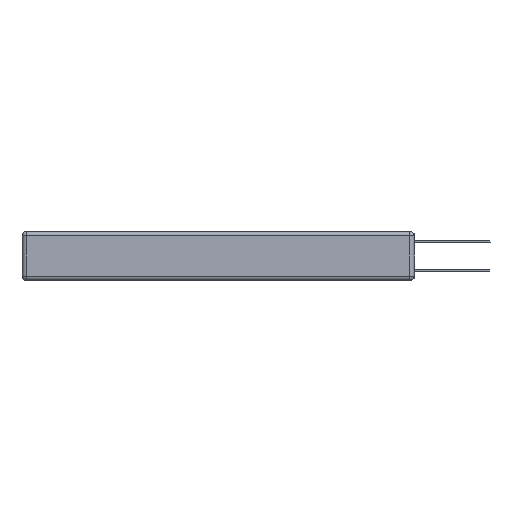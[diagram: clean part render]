
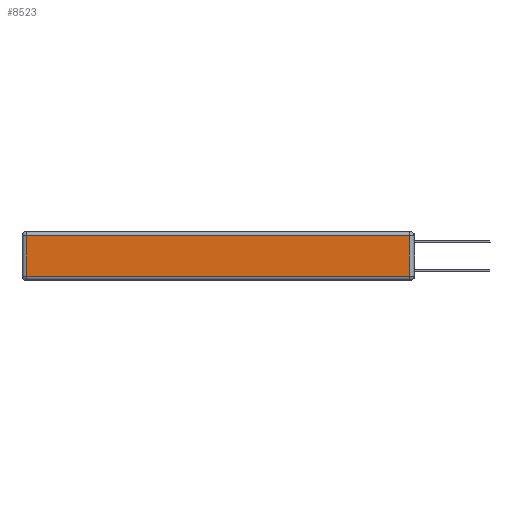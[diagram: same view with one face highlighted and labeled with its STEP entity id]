
A CAD part, left-side view. The second image highlights one B-rep face of the part: STEP entity #8523.
In plain terms, the highlighted planar face has unit normal (-1, 0, 0).
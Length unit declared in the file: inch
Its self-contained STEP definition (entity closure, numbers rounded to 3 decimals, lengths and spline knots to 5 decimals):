
#39 = CARTESIAN_POINT ( 'NONE',  ( 0., 2.72, -0.343 ) ) ;
#441 = VERTEX_POINT ( 'NONE', #12251 ) ;
#1018 = EDGE_CURVE ( 'NONE', #9806, #441, #3056, .T. ) ;
#1954 = EDGE_CURVE ( 'NONE', #6911, #9806, #15482, .T. ) ;
#2604 = VERTEX_POINT ( 'NONE', #8026 ) ;
#2969 = AXIS2_PLACEMENT_3D ( 'NONE', #7080, #16449, #4146 ) ;
#3013 = LINE ( 'NONE', #39, #12522 ) ;
#3056 = LINE ( 'NONE', #7156, #10019 ) ;
#4146 = DIRECTION ( 'NONE',  ( 0., 0., 1. ) ) ;
#5275 = CARTESIAN_POINT ( 'NONE',  ( 0., 0.03, -0.313 ) ) ;
#5506 = EDGE_CURVE ( 'NONE', #2604, #6911, #10618, .T. ) ;
#6911 = VERTEX_POINT ( 'NONE', #5275 ) ;
#7080 = CARTESIAN_POINT ( 'NONE',  ( 0., 0., -0.343 ) ) ;
#7134 = ORIENTED_EDGE ( 'NONE', *, *, #1018, .T. ) ;
#7156 = CARTESIAN_POINT ( 'NONE',  ( 0., 2.75, -0.03 ) ) ;
#7287 = VECTOR ( 'NONE', #13670, 39.37008 ) ;
#8026 = CARTESIAN_POINT ( 'NONE',  ( 0., 2.72, -0.313 ) ) ;
#8049 = FACE_OUTER_BOUND ( 'NONE', #12428, .T. ) ;
#8523 = ADVANCED_FACE ( 'NONE', ( #8049 ), #12398, .T. ) ;
#8541 = ORIENTED_EDGE ( 'NONE', *, *, #5506, .T. ) ;
#8625 = CARTESIAN_POINT ( 'NONE',  ( 0., 0.03, -0.343 ) ) ;
#9091 = CARTESIAN_POINT ( 'NONE',  ( 0., 0.03, -0.03 ) ) ;
#9806 = VERTEX_POINT ( 'NONE', #9091 ) ;
#10019 = VECTOR ( 'NONE', #12945, 39.37008 ) ;
#10618 = LINE ( 'NONE', #17646, #7287 ) ;
#10928 = ORIENTED_EDGE ( 'NONE', *, *, #13962, .T. ) ;
#12251 = CARTESIAN_POINT ( 'NONE',  ( 0., 2.72, -0.03 ) ) ;
#12305 = ORIENTED_EDGE ( 'NONE', *, *, #1954, .T. ) ;
#12398 = PLANE ( 'NONE',  #2969 ) ;
#12428 = EDGE_LOOP ( 'NONE', ( #8541, #12305, #7134, #10928 ) ) ;
#12522 = VECTOR ( 'NONE', #14143, 39.37008 ) ;
#12945 = DIRECTION ( 'NONE',  ( 0., 1., 0. ) ) ;
#13670 = DIRECTION ( 'NONE',  ( 0., -1., 0. ) ) ;
#13962 = EDGE_CURVE ( 'NONE', #441, #2604, #3013, .T. ) ;
#14127 = DIRECTION ( 'NONE',  ( 0., 0., 1. ) ) ;
#14143 = DIRECTION ( 'NONE',  ( 0., 0., -1. ) ) ;
#15482 = LINE ( 'NONE', #8625, #15849 ) ;
#15849 = VECTOR ( 'NONE', #14127, 39.37008 ) ;
#16449 = DIRECTION ( 'NONE',  ( -1., 0., 0. ) ) ;
#17646 = CARTESIAN_POINT ( 'NONE',  ( 0., 0., -0.313 ) ) ;
